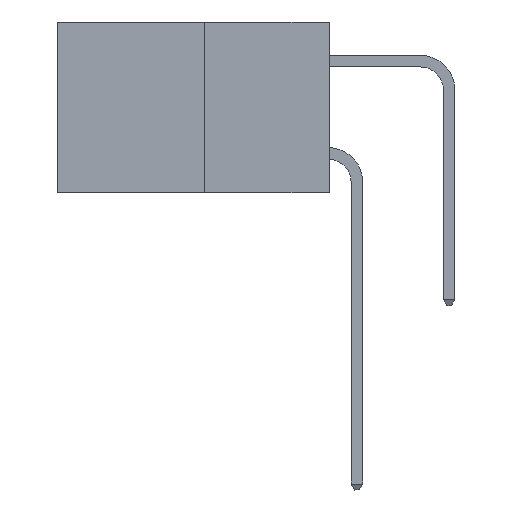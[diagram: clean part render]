
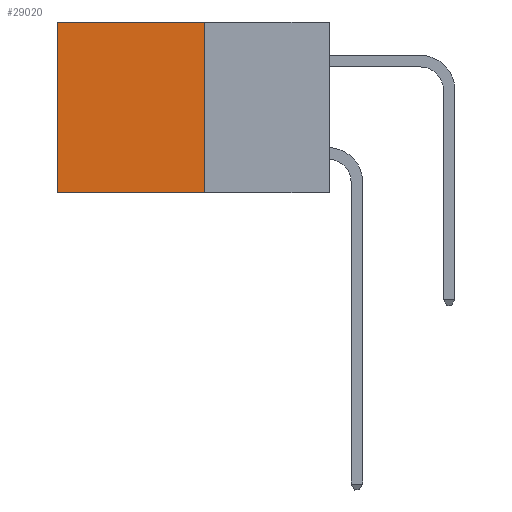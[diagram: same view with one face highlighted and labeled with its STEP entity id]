
A CAD part, left-side view. The second image highlights one B-rep face of the part: STEP entity #29020.
In plain terms, the highlighted planar face has unit normal (-1, 0, 0).
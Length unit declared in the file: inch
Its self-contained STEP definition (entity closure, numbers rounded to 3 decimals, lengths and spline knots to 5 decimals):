
#423 = VECTOR ( 'NONE', #31047, 39.37008 ) ;
#1204 = EDGE_LOOP ( 'NONE', ( #2513, #29398, #27194, #4326 ) ) ;
#2513 = ORIENTED_EDGE ( 'NONE', *, *, #18626, .T. ) ;
#4326 = ORIENTED_EDGE ( 'NONE', *, *, #14347, .T. ) ;
#5309 = CARTESIAN_POINT ( 'NONE',  ( 0.277, 0.27, -0.37 ) ) ;
#6240 = LINE ( 'NONE', #18392, #25776 ) ;
#7014 = VECTOR ( 'NONE', #20837, 39.37008 ) ;
#13302 = VERTEX_POINT ( 'NONE', #24510 ) ;
#13625 = CARTESIAN_POINT ( 'NONE',  ( 0.277, 0.59, -0.37 ) ) ;
#13697 = VERTEX_POINT ( 'NONE', #20827 ) ;
#14347 = EDGE_CURVE ( 'NONE', #13302, #13697, #20832, .T. ) ;
#14792 = DIRECTION ( 'NONE',  ( 1., 0., 0. ) ) ;
#15419 = LINE ( 'NONE', #5309, #28961 ) ;
#15798 = DIRECTION ( 'NONE',  ( 0., 0., -1. ) ) ;
#18274 = CARTESIAN_POINT ( 'NONE',  ( 0.277, 0.59, -0.37 ) ) ;
#18392 = CARTESIAN_POINT ( 'NONE',  ( 0.277, 0.27, -0.37 ) ) ;
#18594 = EDGE_CURVE ( 'NONE', #20961, #28019, #15419, .T. ) ;
#18626 = EDGE_CURVE ( 'NONE', #13697, #28019, #27379, .T. ) ;
#18667 = EDGE_CURVE ( 'NONE', #13302, #20961, #6240, .T. ) ;
#19663 = FACE_OUTER_BOUND ( 'NONE', #1204, .T. ) ;
#20827 = CARTESIAN_POINT ( 'NONE',  ( 0.277, 0.59, 0. ) ) ;
#20832 = LINE ( 'NONE', #28540, #423 ) ;
#20837 = DIRECTION ( 'NONE',  ( 0., 0., -1. ) ) ;
#20961 = VERTEX_POINT ( 'NONE', #22982 ) ;
#22887 = AXIS2_PLACEMENT_3D ( 'NONE', #30008, #14792, #32533 ) ;
#22982 = CARTESIAN_POINT ( 'NONE',  ( 0.277, 0.27, -0.37 ) ) ;
#24510 = CARTESIAN_POINT ( 'NONE',  ( 0.277, 0.27, 0. ) ) ;
#24950 = PLANE ( 'NONE',  #22887 ) ;
#25776 = VECTOR ( 'NONE', #15798, 39.37008 ) ;
#27194 = ORIENTED_EDGE ( 'NONE', *, *, #18667, .F. ) ;
#27379 = LINE ( 'NONE', #18274, #7014 ) ;
#28019 = VERTEX_POINT ( 'NONE', #13625 ) ;
#28280 = DIRECTION ( 'NONE',  ( 0., 1., 0. ) ) ;
#28540 = CARTESIAN_POINT ( 'NONE',  ( 0.277, 0.27, 0. ) ) ;
#28961 = VECTOR ( 'NONE', #28280, 39.37008 ) ;
#29020 = ADVANCED_FACE ( 'NONE', ( #19663 ), #24950, .F. ) ;
#29398 = ORIENTED_EDGE ( 'NONE', *, *, #18594, .F. ) ;
#30008 = CARTESIAN_POINT ( 'NONE',  ( 0.277, 0.27, -0.37 ) ) ;
#31047 = DIRECTION ( 'NONE',  ( 0., 1., 0. ) ) ;
#32533 = DIRECTION ( 'NONE',  ( 0., 0., -1. ) ) ;
